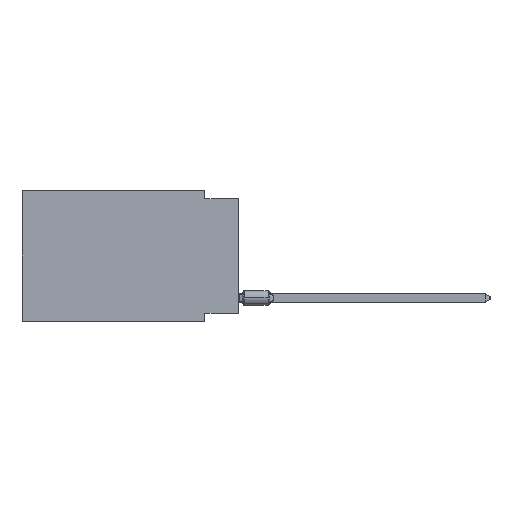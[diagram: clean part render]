
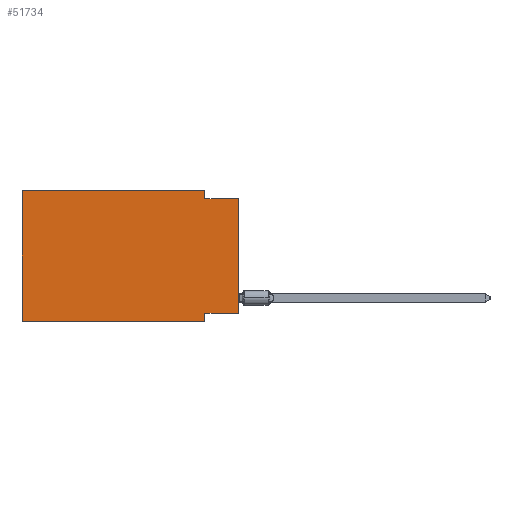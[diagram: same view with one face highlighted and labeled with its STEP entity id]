
A CAD part, left-side view. The second image highlights one B-rep face of the part: STEP entity #51734.
In plain terms, the highlighted planar face has unit normal (-1, 0, 0).
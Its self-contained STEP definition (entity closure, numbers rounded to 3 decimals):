
#2732 = EDGE_CURVE ( 'NONE', #69310, #30178, #48898, .T. ) ;
#5326 = VERTEX_POINT ( 'NONE', #58191 ) ;
#6060 = DIRECTION ( 'NONE',  ( 0., -1., 0. ) ) ;
#8560 = ORIENTED_EDGE ( 'NONE', *, *, #62319, .T. ) ;
#9036 = CARTESIAN_POINT ( 'NONE',  ( 0., 2.54, -9.271 ) ) ;
#10812 = ORIENTED_EDGE ( 'NONE', *, *, #65821, .F. ) ;
#11276 = CARTESIAN_POINT ( 'NONE',  ( 0., 2.54, 0. ) ) ;
#11444 = CARTESIAN_POINT ( 'NONE',  ( 0., 2.54, 0. ) ) ;
#11742 = VECTOR ( 'NONE', #31394, 1000. ) ;
#12502 = EDGE_CURVE ( 'NONE', #40892, #64364, #61081, .T. ) ;
#13438 = ORIENTED_EDGE ( 'NONE', *, *, #12502, .F. ) ;
#19228 = DIRECTION ( 'NONE',  ( 0., 0., -1. ) ) ;
#20119 = DIRECTION ( 'NONE',  ( 0., 0., 1. ) ) ;
#22243 = VERTEX_POINT ( 'NONE', #34079 ) ;
#25220 = ORIENTED_EDGE ( 'NONE', *, *, #74135, .F. ) ;
#27068 = EDGE_CURVE ( 'NONE', #64364, #5326, #66068, .T. ) ;
#27547 = VECTOR ( 'NONE', #20119, 1000. ) ;
#27974 = CARTESIAN_POINT ( 'NONE',  ( 0., 16.383, 0. ) ) ;
#30178 = VERTEX_POINT ( 'NONE', #11276 ) ;
#30180 = CARTESIAN_POINT ( 'NONE',  ( 0., 16.383, 0. ) ) ;
#30279 = VECTOR ( 'NONE', #6060, 1000. ) ;
#30413 = AXIS2_PLACEMENT_3D ( 'NONE', #50361, #68364, #62099 ) ;
#31173 = LINE ( 'NONE', #37791, #46285 ) ;
#31394 = DIRECTION ( 'NONE',  ( 0., 1., 0. ) ) ;
#32024 = FACE_OUTER_BOUND ( 'NONE', #49937, .T. ) ;
#32948 = CARTESIAN_POINT ( 'NONE',  ( 0., 16.383, 0. ) ) ;
#33224 = VECTOR ( 'NONE', #36371, 1000. ) ;
#33438 = VERTEX_POINT ( 'NONE', #35971 ) ;
#34079 = CARTESIAN_POINT ( 'NONE',  ( 0., 16.383, -9.906 ) ) ;
#34846 = LINE ( 'NONE', #11444, #67820 ) ;
#35971 = CARTESIAN_POINT ( 'NONE',  ( 0., 0., -0.635 ) ) ;
#36371 = DIRECTION ( 'NONE',  ( 0., -1., 0. ) ) ;
#37413 = DIRECTION ( 'NONE',  ( 0., 0., 1. ) ) ;
#37435 = CARTESIAN_POINT ( 'NONE',  ( 0., 16.383, -9.906 ) ) ;
#37791 = CARTESIAN_POINT ( 'NONE',  ( 0., 0., 0. ) ) ;
#37816 = DIRECTION ( 'NONE',  ( 0., -1., 0. ) ) ;
#39045 = PLANE ( 'NONE',  #30413 ) ;
#40892 = VERTEX_POINT ( 'NONE', #72589 ) ;
#41432 = CARTESIAN_POINT ( 'NONE',  ( 0., 2.54, -9.906 ) ) ;
#42605 = CARTESIAN_POINT ( 'NONE',  ( 0., 0., -0.635 ) ) ;
#43595 = VERTEX_POINT ( 'NONE', #60129 ) ;
#46285 = VECTOR ( 'NONE', #37413, 1000. ) ;
#46297 = EDGE_CURVE ( 'NONE', #22243, #69310, #61861, .T. ) ;
#47304 = DIRECTION ( 'NONE',  ( 0., 0., -1. ) ) ;
#48898 = LINE ( 'NONE', #30180, #30279 ) ;
#49527 = LINE ( 'NONE', #37435, #59036 ) ;
#49937 = EDGE_LOOP ( 'NONE', ( #58554, #10812, #25220, #70261, #60788, #8560, #61272, #13438 ) ) ;
#50361 = CARTESIAN_POINT ( 'NONE',  ( 0., 16.383, 0. ) ) ;
#51734 = ADVANCED_FACE ( 'NONE', ( #32024 ), #39045, .F. ) ;
#54823 = CARTESIAN_POINT ( 'NONE',  ( 0., 0., -9.271 ) ) ;
#55941 = VECTOR ( 'NONE', #19228, 1000. ) ;
#58191 = CARTESIAN_POINT ( 'NONE',  ( 0., 2.54, -9.906 ) ) ;
#58554 = ORIENTED_EDGE ( 'NONE', *, *, #60054, .T. ) ;
#59036 = VECTOR ( 'NONE', #37816, 1000. ) ;
#59797 = LINE ( 'NONE', #42605, #33224 ) ;
#60054 = EDGE_CURVE ( 'NONE', #40892, #33438, #31173, .T. ) ;
#60129 = CARTESIAN_POINT ( 'NONE',  ( 0., 2.54, -0.635 ) ) ;
#60788 = ORIENTED_EDGE ( 'NONE', *, *, #46297, .F. ) ;
#61081 = LINE ( 'NONE', #54823, #11742 ) ;
#61272 = ORIENTED_EDGE ( 'NONE', *, *, #27068, .F. ) ;
#61861 = LINE ( 'NONE', #32948, #27547 ) ;
#62099 = DIRECTION ( 'NONE',  ( 0., 0., -1. ) ) ;
#62319 = EDGE_CURVE ( 'NONE', #22243, #5326, #49527, .T. ) ;
#64364 = VERTEX_POINT ( 'NONE', #9036 ) ;
#65821 = EDGE_CURVE ( 'NONE', #43595, #33438, #59797, .T. ) ;
#66068 = LINE ( 'NONE', #41432, #55941 ) ;
#67820 = VECTOR ( 'NONE', #47304, 1000. ) ;
#68364 = DIRECTION ( 'NONE',  ( 1., 0., 0. ) ) ;
#69310 = VERTEX_POINT ( 'NONE', #27974 ) ;
#70261 = ORIENTED_EDGE ( 'NONE', *, *, #2732, .F. ) ;
#72589 = CARTESIAN_POINT ( 'NONE',  ( 0., 0., -9.271 ) ) ;
#74135 = EDGE_CURVE ( 'NONE', #30178, #43595, #34846, .T. ) ;
